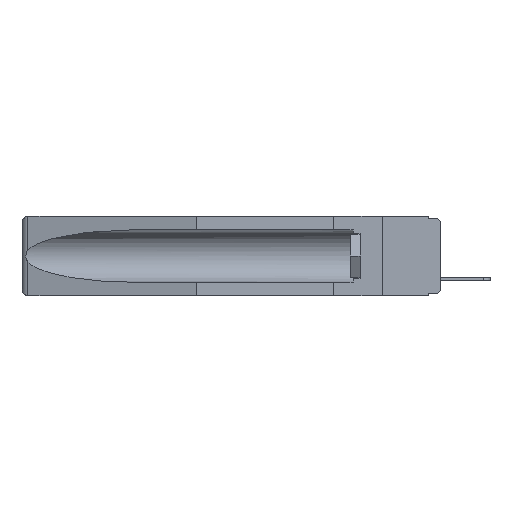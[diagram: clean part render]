
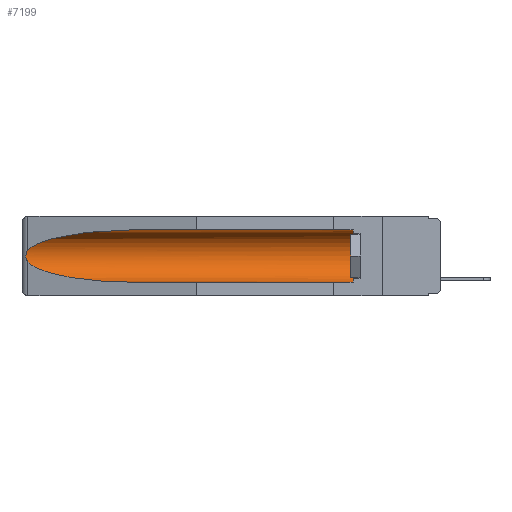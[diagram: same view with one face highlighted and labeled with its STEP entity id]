
A CAD part, left-side view. The second image highlights one B-rep face of the part: STEP entity #7199.
In plain terms, the highlighted cylindrical face has radius 2.857 mm (diameter 5.715 mm), a partial arc.
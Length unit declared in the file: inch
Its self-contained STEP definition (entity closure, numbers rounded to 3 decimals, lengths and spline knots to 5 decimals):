
#1157 = ORIENTED_EDGE ( 'NONE', *, *, #20495, .T. ) ;
#1197 = ORIENTED_EDGE ( 'NONE', *, *, #2915, .T. ) ;
#1233 = CARTESIAN_POINT ( 'NONE',  ( 0.155, 0.126, -0.059 ) ) ;
#1772 = CARTESIAN_POINT ( 'NONE',  ( 0.26597, 1.5296, -0.19026 ) ) ;
#1927 = DIRECTION ( 'NONE',  ( 0., 1., 0. ) ) ;
#2206 = EDGE_CURVE ( 'NONE', #11367, #9381, #18474, .T. ) ;
#2915 = EDGE_CURVE ( 'NONE', #21355, #17140, #14064, .T. ) ;
#3048 = CARTESIAN_POINT ( 'NONE',  ( 0.26537, 1.52718, -0.14972 ) ) ;
#3210 = VECTOR ( 'NONE', #16891, 39.37008 ) ;
#3216 = CARTESIAN_POINT ( 'NONE',  ( 0.26654, 1.53092, -0.15636 ) ) ;
#3346 = CARTESIAN_POINT ( 'NONE',  ( 0.155, 1.07973, -0.059 ) ) ;
#4236 = ORIENTED_EDGE ( 'NONE', *, *, #2206, .T. ) ;
#5198 = CARTESIAN_POINT ( 'NONE',  ( 0.26537, 1.52718, -0.19328 ) ) ;
#6086 = DIRECTION ( 'NONE',  ( 0., 0., 1. ) ) ;
#6281 =( BOUNDED_CURVE ( )  B_SPLINE_CURVE ( 3, ( #3346, #20633, #18811, #22347 ),
 .UNSPECIFIED., .F., .F. ) 
 B_SPLINE_CURVE_WITH_KNOTS ( ( 4, 4 ),
 ( 4.71239, 6.08839 ),
 .UNSPECIFIED. ) 
 CURVE ( )  GEOMETRIC_REPRESENTATION_ITEM ( )  RATIONAL_B_SPLINE_CURVE ( ( 1., 0.848, 0.848, 1. ) ) 
 REPRESENTATION_ITEM ( '' )  );
#6862 = CARTESIAN_POINT ( 'NONE',  ( 0.2673, 1.53269, -0.17917 ) ) ;
#7199 = ADVANCED_FACE ( 'NONE', ( #13501 ), #11832, .F. ) ;
#7556 = CARTESIAN_POINT ( 'NONE',  ( 0.155, 1.07973, -0.284 ) ) ;
#7560 = EDGE_CURVE ( 'NONE', #9381, #10785, #9375, .T. ) ;
#7623 = CARTESIAN_POINT ( 'NONE',  ( 0.26537, 1.52718, -0.19328 ) ) ;
#7638 = EDGE_CURVE ( 'NONE', #11367, #17140, #10483, .T. ) ;
#7811 = CARTESIAN_POINT ( 'NONE',  ( 0.155, 1.07973, -0.059 ) ) ;
#8825 = CARTESIAN_POINT ( 'NONE',  ( 0.155, -0.30754, -0.284 ) ) ;
#9375 = LINE ( 'NONE', #18382, #3210 ) ;
#9381 = VERTEX_POINT ( 'NONE', #1233 ) ;
#9390 = EDGE_LOOP ( 'NONE', ( #1157, #21440, #1197, #20344, #4236, #21744 ) ) ;
#10013 = B_SPLINE_CURVE_WITH_KNOTS ( 'NONE', 3,
 ( #22220, #13552, #3216, #10198, #13699, #15513, #6862, #10340, #1772, #15442 ),
 .UNSPECIFIED., .F., .F.,
 ( 4, 2, 2, 2, 4 ),
 ( 0., 0.00029, 0.00058, 0.00087, 0.00117 ),
 .UNSPECIFIED. ) ;
#10198 = CARTESIAN_POINT ( 'NONE',  ( 0.2673, 1.5327, -0.16383 ) ) ;
#10340 = CARTESIAN_POINT ( 'NONE',  ( 0.26655, 1.53094, -0.18657 ) ) ;
#10483 = LINE ( 'NONE', #8825, #13732 ) ;
#10785 = VERTEX_POINT ( 'NONE', #7811 ) ;
#11192 = CARTESIAN_POINT ( 'NONE',  ( 0.21114, 1.30732, -0.284 ) ) ;
#11303 = CARTESIAN_POINT ( 'NONE',  ( 0.155, 0.126, -0.1715 ) ) ;
#11367 = VERTEX_POINT ( 'NONE', #16744 ) ;
#11435 = CARTESIAN_POINT ( 'NONE',  ( 0.155, 1.07973, -0.284 ) ) ;
#11832 = CYLINDRICAL_SURFACE ( 'NONE', #21895, 0.1125 ) ;
#13084 = EDGE_CURVE ( 'NONE', #16081, #21355, #10013, .T. ) ;
#13501 = FACE_OUTER_BOUND ( 'NONE', #9390, .T. ) ;
#13518 = CARTESIAN_POINT ( 'NONE',  ( 0.155, -0.30754, -0.1715 ) ) ;
#13552 = CARTESIAN_POINT ( 'NONE',  ( 0.26597, 1.52961, -0.15275 ) ) ;
#13699 = CARTESIAN_POINT ( 'NONE',  ( 0.2675, 1.53308, -0.16763 ) ) ;
#13732 = VECTOR ( 'NONE', #1927, 39.37008 ) ;
#14064 =( BOUNDED_CURVE ( )  B_SPLINE_CURVE ( 3, ( #7623, #21545, #11192, #7556 ),
 .UNSPECIFIED., .F., .F. ) 
 B_SPLINE_CURVE_WITH_KNOTS ( ( 4, 4 ),
 ( 0.1948, 1.5708 ),
 .UNSPECIFIED. ) 
 CURVE ( )  GEOMETRIC_REPRESENTATION_ITEM ( )  RATIONAL_B_SPLINE_CURVE ( ( 1., 0.848, 0.848, 1. ) ) 
 REPRESENTATION_ITEM ( '' )  );
#15191 = AXIS2_PLACEMENT_3D ( 'NONE', #11303, #21585, #6086 ) ;
#15442 = CARTESIAN_POINT ( 'NONE',  ( 0.26537, 1.52718, -0.19328 ) ) ;
#15513 = CARTESIAN_POINT ( 'NONE',  ( 0.2675, 1.53308, -0.17534 ) ) ;
#16081 = VERTEX_POINT ( 'NONE', #3048 ) ;
#16744 = CARTESIAN_POINT ( 'NONE',  ( 0.155, 0.126, -0.284 ) ) ;
#16891 = DIRECTION ( 'NONE',  ( 0., 1., 0. ) ) ;
#17140 = VERTEX_POINT ( 'NONE', #11435 ) ;
#18382 = CARTESIAN_POINT ( 'NONE',  ( 0.155, -0.30754, -0.059 ) ) ;
#18474 = CIRCLE ( 'NONE', #15191, 0.1125 ) ;
#18811 = CARTESIAN_POINT ( 'NONE',  ( 0.25451, 1.48313, -0.09465 ) ) ;
#18950 = DIRECTION ( 'NONE',  ( 0., 0., 1. ) ) ;
#20344 = ORIENTED_EDGE ( 'NONE', *, *, #7638, .F. ) ;
#20495 = EDGE_CURVE ( 'NONE', #10785, #16081, #6281, .T. ) ;
#20544 = DIRECTION ( 'NONE',  ( 0., 1., 0. ) ) ;
#20633 = CARTESIAN_POINT ( 'NONE',  ( 0.21114, 1.30732, -0.059 ) ) ;
#21355 = VERTEX_POINT ( 'NONE', #5198 ) ;
#21440 = ORIENTED_EDGE ( 'NONE', *, *, #13084, .T. ) ;
#21545 = CARTESIAN_POINT ( 'NONE',  ( 0.25451, 1.48313, -0.24835 ) ) ;
#21585 = DIRECTION ( 'NONE',  ( 0., -1., 0. ) ) ;
#21744 = ORIENTED_EDGE ( 'NONE', *, *, #7560, .T. ) ;
#21895 = AXIS2_PLACEMENT_3D ( 'NONE', #13518, #20544, #18950 ) ;
#22220 = CARTESIAN_POINT ( 'NONE',  ( 0.26537, 1.52718, -0.14972 ) ) ;
#22347 = CARTESIAN_POINT ( 'NONE',  ( 0.26537, 1.52718, -0.14972 ) ) ;
